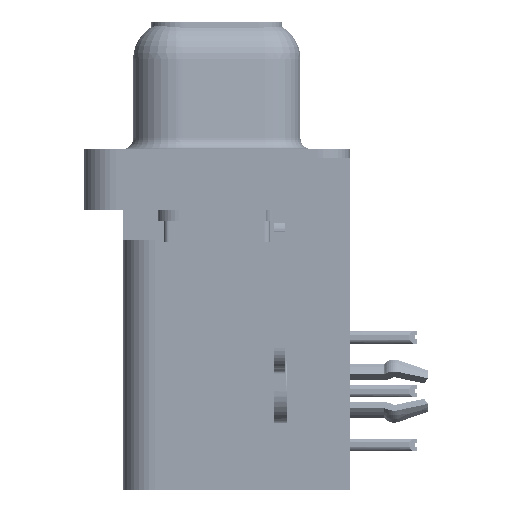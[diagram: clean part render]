
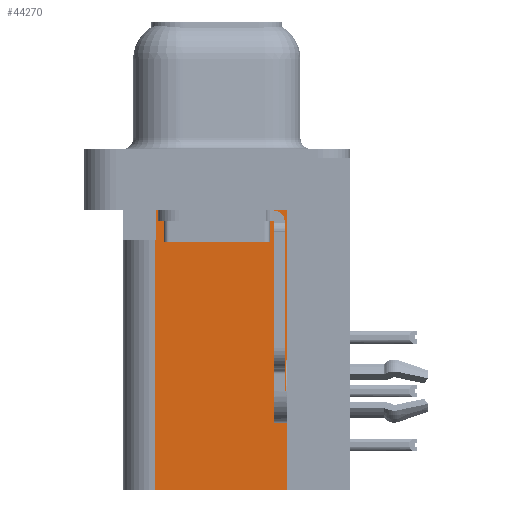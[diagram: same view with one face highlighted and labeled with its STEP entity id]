
A CAD part, left-side view. The second image highlights one B-rep face of the part: STEP entity #44270.
In plain terms, the highlighted planar face has unit normal (-1, 0, 0).
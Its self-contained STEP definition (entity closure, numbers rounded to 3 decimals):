
#349 = DIRECTION ( 'NONE',  ( 0., 0., 1. ) ) ;
#391 = VECTOR ( 'NONE', #26467, 1000. ) ;
#428 = LINE ( 'NONE', #29769, #391 ) ;
#1033 = EDGE_CURVE ( 'NONE', #26580, #29794, #28320, .T. ) ;
#1567 = VECTOR ( 'NONE', #349, 1000. ) ;
#1755 = LINE ( 'NONE', #14560, #1567 ) ;
#1818 = ORIENTED_EDGE ( 'NONE', *, *, #17638, .F. ) ;
#1830 = CARTESIAN_POINT ( 'NONE',  ( 3.7, -3.295, -2.5 ) ) ;
#3053 = FACE_OUTER_BOUND ( 'NONE', #13945, .T. ) ;
#3087 = CARTESIAN_POINT ( 'NONE',  ( 3.7, 2.925, -15.7 ) ) ;
#3264 = EDGE_CURVE ( 'NONE', #29794, #20993, #27995, .T. ) ;
#3643 = CARTESIAN_POINT ( 'NONE',  ( 3.7, -3.295, -15.7 ) ) ;
#4040 = VECTOR ( 'NONE', #42960, 1000. ) ;
#4287 = LINE ( 'NONE', #3643, #4040 ) ;
#5612 = EDGE_CURVE ( 'NONE', #20993, #40011, #23516, .T. ) ;
#9684 = DIRECTION ( 'NONE',  ( 1., 0., 0. ) ) ;
#10105 = CARTESIAN_POINT ( 'NONE',  ( 3.7, 2.925, -3.9 ) ) ;
#10133 = ORIENTED_EDGE ( 'NONE', *, *, #5612, .T. ) ;
#10358 = DIRECTION ( 'NONE',  ( 0., 1., 0. ) ) ;
#10833 = CARTESIAN_POINT ( 'NONE',  ( 3.7, -3.295, -15.7 ) ) ;
#11160 = VERTEX_POINT ( 'NONE', #3087 ) ;
#13797 = DIRECTION ( 'NONE',  ( 0., 0., -1. ) ) ;
#13945 = EDGE_LOOP ( 'NONE', ( #42501, #18083, #10133, #1818, #28511, #17100 ) ) ;
#14560 = CARTESIAN_POINT ( 'NONE',  ( 3.7, 2.925, -15.7 ) ) ;
#16575 = CARTESIAN_POINT ( 'NONE',  ( 3.7, 2.895, -3.9 ) ) ;
#17100 = ORIENTED_EDGE ( 'NONE', *, *, #20161, .T. ) ;
#17638 = EDGE_CURVE ( 'NONE', #11160, #40011, #1755, .T. ) ;
#18083 = ORIENTED_EDGE ( 'NONE', *, *, #3264, .T. ) ;
#19935 = EDGE_CURVE ( 'NONE', #40547, #11160, #4287, .T. ) ;
#20161 = EDGE_CURVE ( 'NONE', #40547, #26580, #428, .T. ) ;
#20993 = VERTEX_POINT ( 'NONE', #16575 ) ;
#23516 = LINE ( 'NONE', #24656, #24037 ) ;
#24037 = VECTOR ( 'NONE', #10358, 1000. ) ;
#24656 = CARTESIAN_POINT ( 'NONE',  ( 3.7, 0., -3.9 ) ) ;
#26467 = DIRECTION ( 'NONE',  ( 0., 0., 1. ) ) ;
#26539 = VECTOR ( 'NONE', #32054, 1000. ) ;
#26580 = VERTEX_POINT ( 'NONE', #39843 ) ;
#27798 = AXIS2_PLACEMENT_3D ( 'NONE', #45858, #9684, #38704 ) ;
#27995 = LINE ( 'NONE', #35339, #28355 ) ;
#28320 = LINE ( 'NONE', #1830, #26539 ) ;
#28355 = VECTOR ( 'NONE', #13797, 1000. ) ;
#28511 = ORIENTED_EDGE ( 'NONE', *, *, #19935, .F. ) ;
#29769 = CARTESIAN_POINT ( 'NONE',  ( 3.7, -3.295, -15.7 ) ) ;
#29794 = VERTEX_POINT ( 'NONE', #37170 ) ;
#31500 = PLANE ( 'NONE',  #27798 ) ;
#32054 = DIRECTION ( 'NONE',  ( 0., 1., 0. ) ) ;
#35339 = CARTESIAN_POINT ( 'NONE',  ( 3.7, 2.895, -3.9 ) ) ;
#37170 = CARTESIAN_POINT ( 'NONE',  ( 3.7, 2.895, -2.5 ) ) ;
#38704 = DIRECTION ( 'NONE',  ( 0., 0., -1. ) ) ;
#39843 = CARTESIAN_POINT ( 'NONE',  ( 3.7, -3.295, -2.5 ) ) ;
#40011 = VERTEX_POINT ( 'NONE', #10105 ) ;
#40547 = VERTEX_POINT ( 'NONE', #10833 ) ;
#42501 = ORIENTED_EDGE ( 'NONE', *, *, #1033, .T. ) ;
#42960 = DIRECTION ( 'NONE',  ( 0., 1., 0. ) ) ;
#44270 = ADVANCED_FACE ( 'NONE', ( #3053 ), #31500, .F. ) ;
#45858 = CARTESIAN_POINT ( 'NONE',  ( 3.7, -3.295, -15.7 ) ) ;
